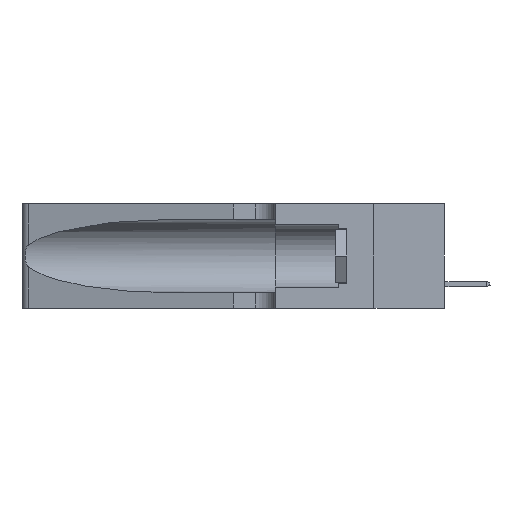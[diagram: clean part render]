
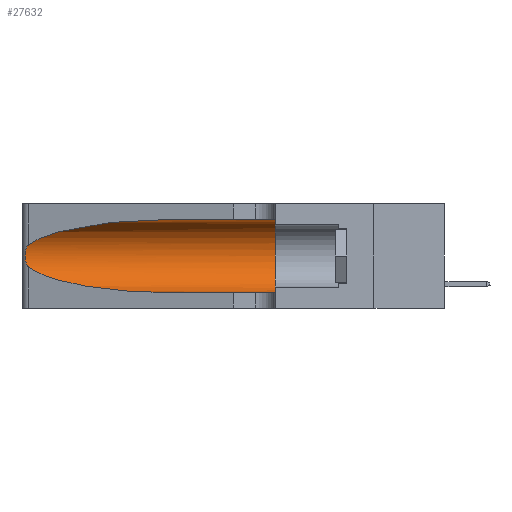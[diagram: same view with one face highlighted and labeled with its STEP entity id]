
A CAD part, left-side view. The second image highlights one B-rep face of the part: STEP entity #27632.
In plain terms, the highlighted cylindrical face has radius 3.308 mm (diameter 6.617 mm), a partial arc.
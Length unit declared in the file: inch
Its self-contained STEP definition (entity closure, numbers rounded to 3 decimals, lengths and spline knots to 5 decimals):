
#175 = DIRECTION ( 'NONE',  ( 0., -1., 0. ) ) ;
#630 = DIRECTION ( 'NONE',  ( 0., 0., -1. ) ) ;
#1348 = DIRECTION ( 'NONE',  ( 0., 1., 0. ) ) ;
#2719 = CARTESIAN_POINT ( 'NONE',  ( 0.1305, 0.72297, 0.31525 ) ) ;
#3391 = B_SPLINE_CURVE_WITH_KNOTS ( 'NONE', 3,
 ( #12444, #12065, #10353, #13196, #12823, #33909, #17070, #34283, #20133, #25795, #9102, #34041, #26394, #24641 ),
 .UNSPECIFIED., .F., .F.,
 ( 4, 2, 2, 2, 2, 2, 4 ),
 ( 0., 0.00027, 0.00053, 0.00107, 0.0016, 0.00187, 0.00214 ),
 .UNSPECIFIED. ) ;
#3413 = CARTESIAN_POINT ( 'NONE',  ( 0.25487, 1.22718, 0.14631 ) ) ;
#4186 = CARTESIAN_POINT ( 'NONE',  ( 0.1305, 0.35, 0.185 ) ) ;
#4873 = VERTEX_POINT ( 'NONE', #13899 ) ;
#5629 = CARTESIAN_POINT ( 'NONE',  ( 0.18966, 0.96281, 0.31525 ) ) ;
#5656 =( BOUNDED_CURVE ( )  B_SPLINE_CURVE ( 3, ( #2719, #5629, #22298, #25127 ),
 .UNSPECIFIED., .F., .F. ) 
 B_SPLINE_CURVE_WITH_KNOTS ( ( 4, 4 ),
 ( 1.5708, 2.84003 ),
 .UNSPECIFIED. ) 
 CURVE ( )  GEOMETRIC_REPRESENTATION_ITEM ( )  RATIONAL_B_SPLINE_CURVE ( ( 1., 0.87, 0.87, 1. ) ) 
 REPRESENTATION_ITEM ( '' )  );
#5920 = ORIENTED_EDGE ( 'NONE', *, *, #36184, .F. ) ;
#7665 = ORIENTED_EDGE ( 'NONE', *, *, #10958, .T. ) ;
#7793 = VERTEX_POINT ( 'NONE', #33791 ) ;
#9102 = CARTESIAN_POINT ( 'NONE',  ( 0.25789, 1.23486, 0.15765 ) ) ;
#10168 = CIRCLE ( 'NONE', #27251, 0.13025 ) ;
#10353 = CARTESIAN_POINT ( 'NONE',  ( 0.25639, 1.23184, 0.21858 ) ) ;
#10370 = CARTESIAN_POINT ( 'NONE',  ( 0.1305, 0.72297, 0.05475 ) ) ;
#10958 = EDGE_CURVE ( 'NONE', #18439, #7793, #3391, .T. ) ;
#11249 = CARTESIAN_POINT ( 'NONE',  ( 0.1305, 0.35, 0.05475 ) ) ;
#12065 = CARTESIAN_POINT ( 'NONE',  ( 0.25555, 1.22994, 0.2215 ) ) ;
#12444 = CARTESIAN_POINT ( 'NONE',  ( 0.25487, 1.22718, 0.22369 ) ) ;
#12823 = CARTESIAN_POINT ( 'NONE',  ( 0.25854, 1.2359, 0.20912 ) ) ;
#13196 = CARTESIAN_POINT ( 'NONE',  ( 0.25787, 1.23484, 0.2124 ) ) ;
#13484 = LINE ( 'NONE', #22791, #31012 ) ;
#13899 = CARTESIAN_POINT ( 'NONE',  ( 0.1305, 0.72297, 0.31525 ) ) ;
#14334 = CARTESIAN_POINT ( 'NONE',  ( 0.1305, 0.72297, 0.05475 ) ) ;
#16466 =( BOUNDED_CURVE ( )  B_SPLINE_CURVE ( 3, ( #3413, #23152, #19951, #14334 ),
 .UNSPECIFIED., .F., .F. ) 
 B_SPLINE_CURVE_WITH_KNOTS ( ( 4, 4 ),
 ( 3.44316, 4.71239 ),
 .UNSPECIFIED. ) 
 CURVE ( )  GEOMETRIC_REPRESENTATION_ITEM ( )  RATIONAL_B_SPLINE_CURVE ( ( 1., 0.87, 0.87, 1. ) ) 
 REPRESENTATION_ITEM ( '' )  );
#17070 = CARTESIAN_POINT ( 'NONE',  ( 0.26075, 1.23896, 0.19203 ) ) ;
#17479 = VERTEX_POINT ( 'NONE', #11249 ) ;
#17542 = EDGE_CURVE ( 'NONE', #24162, #17479, #22000, .T. ) ;
#18373 = DIRECTION ( 'NONE',  ( 0., 0., 1. ) ) ;
#18439 = VERTEX_POINT ( 'NONE', #31584 ) ;
#19935 = EDGE_CURVE ( 'NONE', #4873, #33975, #13484, .T. ) ;
#19951 = CARTESIAN_POINT ( 'NONE',  ( 0.18966, 0.96281, 0.05475 ) ) ;
#20133 = CARTESIAN_POINT ( 'NONE',  ( 0.26017, 1.23833, 0.17102 ) ) ;
#20419 = AXIS2_PLACEMENT_3D ( 'NONE', #22688, #175, #630 ) ;
#20732 = ORIENTED_EDGE ( 'NONE', *, *, #19935, .F. ) ;
#21017 = ORIENTED_EDGE ( 'NONE', *, *, #17542, .T. ) ;
#21546 = EDGE_CURVE ( 'NONE', #7793, #24162, #16466, .T. ) ;
#22000 = LINE ( 'NONE', #29022, #22441 ) ;
#22298 = CARTESIAN_POINT ( 'NONE',  ( 0.2373, 1.15595, 0.28018 ) ) ;
#22441 = VECTOR ( 'NONE', #34329, 39.37008 ) ;
#22688 = CARTESIAN_POINT ( 'NONE',  ( 0.1305, 1.61858, 0.185 ) ) ;
#22791 = CARTESIAN_POINT ( 'NONE',  ( 0.1305, 1.61858, 0.31525 ) ) ;
#22924 = DIRECTION ( 'NONE',  ( 0., -1., 0. ) ) ;
#23056 = EDGE_LOOP ( 'NONE', ( #30369, #7665, #24656, #21017, #5920, #20732 ) ) ;
#23152 = CARTESIAN_POINT ( 'NONE',  ( 0.2373, 1.15595, 0.08982 ) ) ;
#24162 = VERTEX_POINT ( 'NONE', #10370 ) ;
#24641 = CARTESIAN_POINT ( 'NONE',  ( 0.25487, 1.22718, 0.14631 ) ) ;
#24656 = ORIENTED_EDGE ( 'NONE', *, *, #21546, .T. ) ;
#25127 = CARTESIAN_POINT ( 'NONE',  ( 0.25487, 1.22718, 0.22369 ) ) ;
#25228 = CARTESIAN_POINT ( 'NONE',  ( 0.1305, 0.35, 0.31525 ) ) ;
#25795 = CARTESIAN_POINT ( 'NONE',  ( 0.25856, 1.23593, 0.16098 ) ) ;
#26394 = CARTESIAN_POINT ( 'NONE',  ( 0.25555, 1.22993, 0.14849 ) ) ;
#27251 = AXIS2_PLACEMENT_3D ( 'NONE', #4186, #1348, #18373 ) ;
#27632 = ADVANCED_FACE ( 'NONE', ( #28827 ), #29762, .F. ) ;
#28238 = EDGE_CURVE ( 'NONE', #4873, #18439, #5656, .T. ) ;
#28827 = FACE_OUTER_BOUND ( 'NONE', #23056, .T. ) ;
#29022 = CARTESIAN_POINT ( 'NONE',  ( 0.1305, 1.61858, 0.05475 ) ) ;
#29762 = CYLINDRICAL_SURFACE ( 'NONE', #20419, 0.13025 ) ;
#30369 = ORIENTED_EDGE ( 'NONE', *, *, #28238, .T. ) ;
#31012 = VECTOR ( 'NONE', #22924, 39.37008 ) ;
#31584 = CARTESIAN_POINT ( 'NONE',  ( 0.25487, 1.22718, 0.22369 ) ) ;
#33791 = CARTESIAN_POINT ( 'NONE',  ( 0.25487, 1.22718, 0.14631 ) ) ;
#33909 = CARTESIAN_POINT ( 'NONE',  ( 0.26018, 1.23835, 0.19895 ) ) ;
#33975 = VERTEX_POINT ( 'NONE', #25228 ) ;
#34041 = CARTESIAN_POINT ( 'NONE',  ( 0.25639, 1.23186, 0.15144 ) ) ;
#34283 = CARTESIAN_POINT ( 'NONE',  ( 0.26075, 1.23896, 0.178 ) ) ;
#34329 = DIRECTION ( 'NONE',  ( 0., -1., 0. ) ) ;
#36184 = EDGE_CURVE ( 'NONE', #33975, #17479, #10168, .T. ) ;
